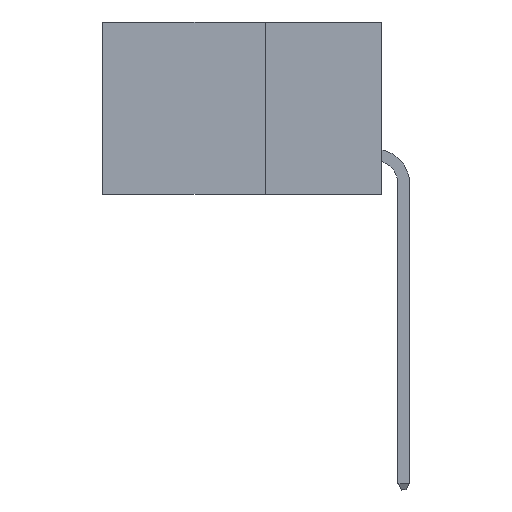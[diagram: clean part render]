
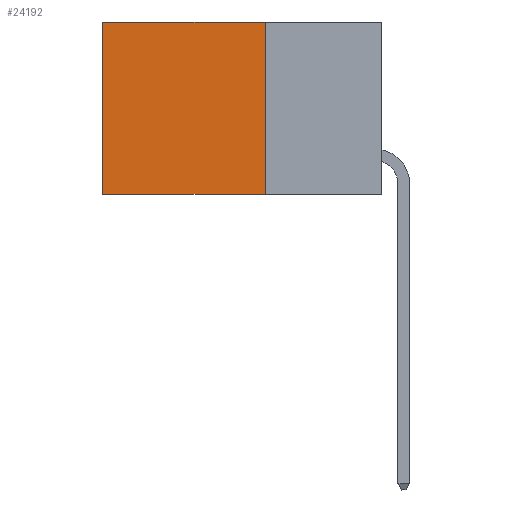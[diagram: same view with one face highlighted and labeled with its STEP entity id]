
A CAD part, left-side view. The second image highlights one B-rep face of the part: STEP entity #24192.
In plain terms, the highlighted planar face has unit normal (-1, 0, 0).
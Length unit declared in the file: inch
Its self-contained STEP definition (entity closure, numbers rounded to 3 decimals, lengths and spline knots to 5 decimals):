
#654 = ORIENTED_EDGE ( 'NONE', *, *, #11339, .F. ) ;
#1156 = EDGE_CURVE ( 'NONE', #20144, #14068, #12100, .T. ) ;
#1283 = VERTEX_POINT ( 'NONE', #14678 ) ;
#1811 = CARTESIAN_POINT ( 'NONE',  ( 0.2875, 0.25, 0. ) ) ;
#1953 = VERTEX_POINT ( 'NONE', #24322 ) ;
#2248 = CARTESIAN_POINT ( 'NONE',  ( 0.2875, 0.6, 0. ) ) ;
#2964 = CARTESIAN_POINT ( 'NONE',  ( 0.2875, 0.25, 0. ) ) ;
#3638 = FACE_OUTER_BOUND ( 'NONE', #5515, .T. ) ;
#4663 = EDGE_CURVE ( 'NONE', #20144, #1283, #15121, .T. ) ;
#5515 = EDGE_LOOP ( 'NONE', ( #11981, #654, #13678, #12978 ) ) ;
#5875 = DIRECTION ( 'NONE',  ( 0., 0., -1. ) ) ;
#6101 = DIRECTION ( 'NONE',  ( 0., 1., 0. ) ) ;
#6239 = VECTOR ( 'NONE', #10279, 39.37008 ) ;
#7776 = VECTOR ( 'NONE', #8410, 39.37008 ) ;
#7993 = VECTOR ( 'NONE', #6101, 39.37008 ) ;
#8410 = DIRECTION ( 'NONE',  ( 0., 0., -1. ) ) ;
#8876 = DIRECTION ( 'NONE',  ( 0., 1., 0. ) ) ;
#9999 = AXIS2_PLACEMENT_3D ( 'NONE', #1811, #15430, #5875 ) ;
#10279 = DIRECTION ( 'NONE',  ( 0., 0., -1. ) ) ;
#11339 = EDGE_CURVE ( 'NONE', #14068, #1953, #16204, .T. ) ;
#11981 = ORIENTED_EDGE ( 'NONE', *, *, #25162, .T. ) ;
#12100 = LINE ( 'NONE', #12225, #7776 ) ;
#12225 = CARTESIAN_POINT ( 'NONE',  ( 0.2875, 0.25, 0. ) ) ;
#12735 = CARTESIAN_POINT ( 'NONE',  ( 0.2875, 0.25, -0.37 ) ) ;
#12978 = ORIENTED_EDGE ( 'NONE', *, *, #4663, .T. ) ;
#13678 = ORIENTED_EDGE ( 'NONE', *, *, #1156, .F. ) ;
#13889 = CARTESIAN_POINT ( 'NONE',  ( 0.2875, 0.25, 0. ) ) ;
#14068 = VERTEX_POINT ( 'NONE', #12735 ) ;
#14678 = CARTESIAN_POINT ( 'NONE',  ( 0.2875, 0.6, 0. ) ) ;
#15121 = LINE ( 'NONE', #2964, #15237 ) ;
#15237 = VECTOR ( 'NONE', #8876, 39.37008 ) ;
#15430 = DIRECTION ( 'NONE',  ( 1., 0., 0. ) ) ;
#16153 = LINE ( 'NONE', #2248, #6239 ) ;
#16204 = LINE ( 'NONE', #23846, #7993 ) ;
#19533 = PLANE ( 'NONE',  #9999 ) ;
#20144 = VERTEX_POINT ( 'NONE', #13889 ) ;
#23846 = CARTESIAN_POINT ( 'NONE',  ( 0.2875, 0.25, -0.37 ) ) ;
#24192 = ADVANCED_FACE ( 'NONE', ( #3638 ), #19533, .F. ) ;
#24322 = CARTESIAN_POINT ( 'NONE',  ( 0.2875, 0.6, -0.37 ) ) ;
#25162 = EDGE_CURVE ( 'NONE', #1283, #1953, #16153, .T. ) ;
